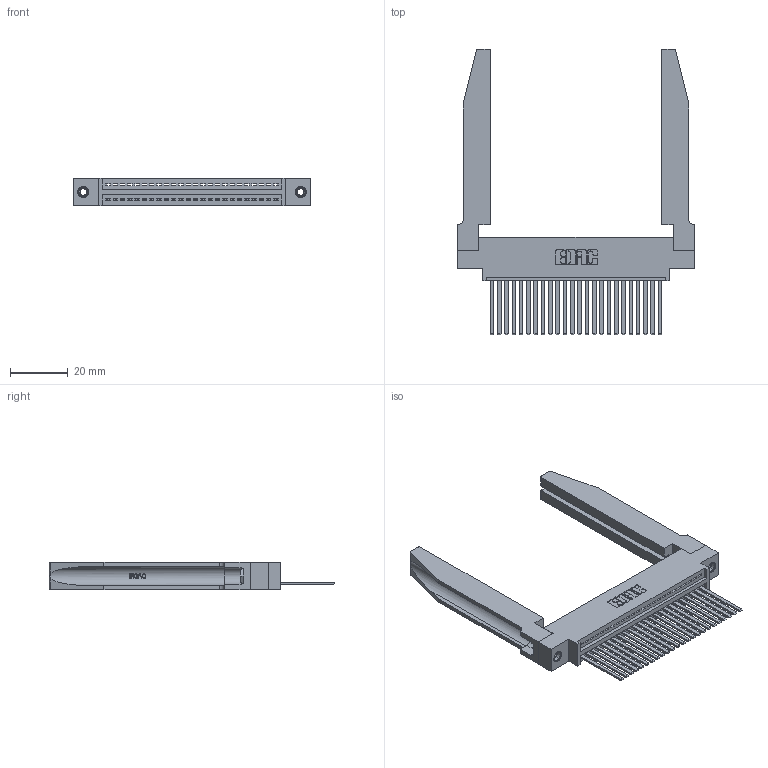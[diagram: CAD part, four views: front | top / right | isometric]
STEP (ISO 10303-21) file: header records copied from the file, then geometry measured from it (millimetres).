
FILE_DESCRIPTION (( 'STEP AP203' ), '1' );
FILE_NAME ('345-024-544-678.STEP', '2019-10-05T05:23:48', ( '' ), ( '' ), 'SwSTEP 2.0', 'SolidWorks 2016', '' );
FILE_SCHEMA (( 'CONFIG_CONTROL_DESIGN' ));
Length unit declared in the file: inch
Products named in the file (5): 345-292-001_345-293-144; 345 Part_0.170 Offset - 0.156 Dia-TH; 345-024-544-678; 345-220-078_345-220-078; 345-250-001_345-250-001-102
Assembly tree (29 placements, depth 2):
  345-024-544-678
    345 Part_0.170 Offset - 0.156 Dia-TH
    345-292-001_345-293-144  x24
    345-250-001_345-250-001-102  x2
    345-220-078_345-220-078  x2
Bounding box: 82.19 x 99.24 x 9.4 mm (x, y, z)
Volume: 15594.5 mm3; surface area: 17959.4 mm2
Topology: 29 solids, 29 shells, 1612 faces, 4753 edges, 3126 vertices
Faces by surface type: plane 1090, cylinder 470, bspline 36, cone 12, torus 4
Entity records: 25174 total; most frequent: CARTESIAN_POINT 5259, ORIENTED_EDGE 4114, DIRECTION 3623, EDGE_CURVE 2057, LINE 1739, VECTOR 1739, VERTEX_POINT 1364, AXIS2_PLACEMENT_3D 942
